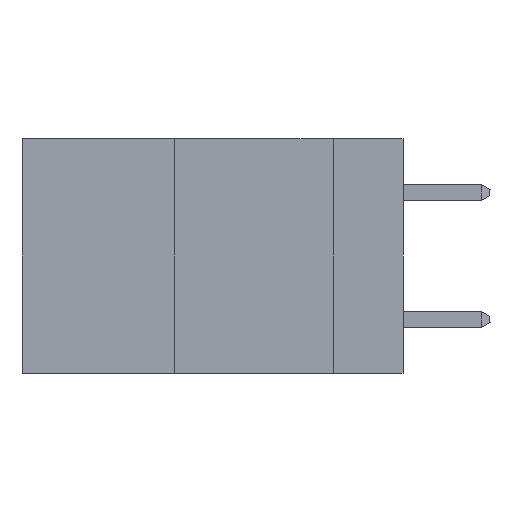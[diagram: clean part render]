
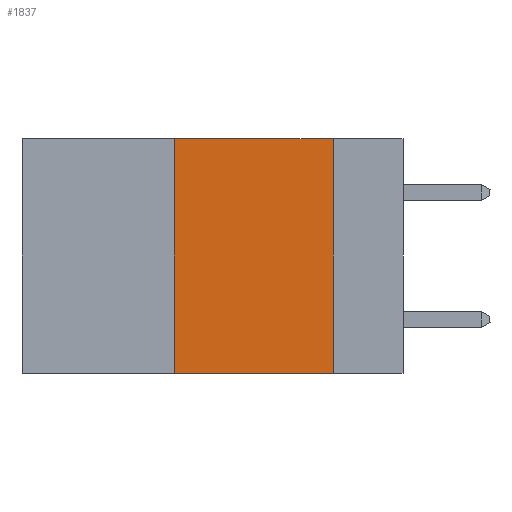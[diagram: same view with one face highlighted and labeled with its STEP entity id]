
A CAD part, left-side view. The second image highlights one B-rep face of the part: STEP entity #1837.
In plain terms, the highlighted planar face has unit normal (-1, 0, 0).
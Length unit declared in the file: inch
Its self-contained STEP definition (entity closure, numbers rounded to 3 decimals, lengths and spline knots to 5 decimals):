
#44 = EDGE_CURVE ( 'NONE', #17141, #4677, #11400, .T. ) ;
#525 = CARTESIAN_POINT ( 'NONE',  ( 0., 0.6, 0. ) ) ;
#1837 = ADVANCED_FACE ( 'NONE', ( #17783 ), #5780, .F. ) ;
#2011 = EDGE_LOOP ( 'NONE', ( #17011, #15035, #6024, #5829 ) ) ;
#2302 = EDGE_CURVE ( 'NONE', #17141, #8834, #4108, .T. ) ;
#2322 = DIRECTION ( 'NONE',  ( 0., 0., -1. ) ) ;
#2368 = DIRECTION ( 'NONE',  ( 0., 0., 1. ) ) ;
#2537 = CARTESIAN_POINT ( 'NONE',  ( 0., 0.36, -0.37 ) ) ;
#4108 = LINE ( 'NONE', #16177, #18023 ) ;
#4677 = VERTEX_POINT ( 'NONE', #11214 ) ;
#5486 = DIRECTION ( 'NONE',  ( 0., -1., 0. ) ) ;
#5780 = PLANE ( 'NONE',  #16419 ) ;
#5829 = ORIENTED_EDGE ( 'NONE', *, *, #44, .T. ) ;
#6024 = ORIENTED_EDGE ( 'NONE', *, *, #2302, .F. ) ;
#6037 = DIRECTION ( 'NONE',  ( 0., 0., -1. ) ) ;
#6354 = CARTESIAN_POINT ( 'NONE',  ( 0., 0.11, 0. ) ) ;
#8174 = CARTESIAN_POINT ( 'NONE',  ( 0., 0.6, -0.37 ) ) ;
#8834 = VERTEX_POINT ( 'NONE', #11190 ) ;
#9003 = CARTESIAN_POINT ( 'NONE',  ( 0., 0.6, 0. ) ) ;
#9142 = DIRECTION ( 'NONE',  ( 1., 0., 0. ) ) ;
#9389 = CARTESIAN_POINT ( 'NONE',  ( 0., 0.11, 0. ) ) ;
#9809 = EDGE_CURVE ( 'NONE', #8834, #14314, #20709, .T. ) ;
#11190 = CARTESIAN_POINT ( 'NONE',  ( 0., 0.36, 0. ) ) ;
#11214 = CARTESIAN_POINT ( 'NONE',  ( 0., 0.11, -0.37 ) ) ;
#11400 = LINE ( 'NONE', #8174, #21002 ) ;
#13349 = DIRECTION ( 'NONE',  ( 0., -1., 0. ) ) ;
#14314 = VERTEX_POINT ( 'NONE', #6354 ) ;
#14383 = VECTOR ( 'NONE', #6037, 39.37008 ) ;
#15035 = ORIENTED_EDGE ( 'NONE', *, *, #9809, .F. ) ;
#16177 = CARTESIAN_POINT ( 'NONE',  ( 0., 0.36, 0. ) ) ;
#16419 = AXIS2_PLACEMENT_3D ( 'NONE', #9003, #9142, #2322 ) ;
#17011 = ORIENTED_EDGE ( 'NONE', *, *, #19512, .F. ) ;
#17141 = VERTEX_POINT ( 'NONE', #2537 ) ;
#17783 = FACE_OUTER_BOUND ( 'NONE', #2011, .T. ) ;
#18023 = VECTOR ( 'NONE', #2368, 39.37008 ) ;
#18408 = LINE ( 'NONE', #9389, #14383 ) ;
#19512 = EDGE_CURVE ( 'NONE', #14314, #4677, #18408, .T. ) ;
#20709 = LINE ( 'NONE', #525, #22024 ) ;
#21002 = VECTOR ( 'NONE', #13349, 39.37008 ) ;
#22024 = VECTOR ( 'NONE', #5486, 39.37008 ) ;
